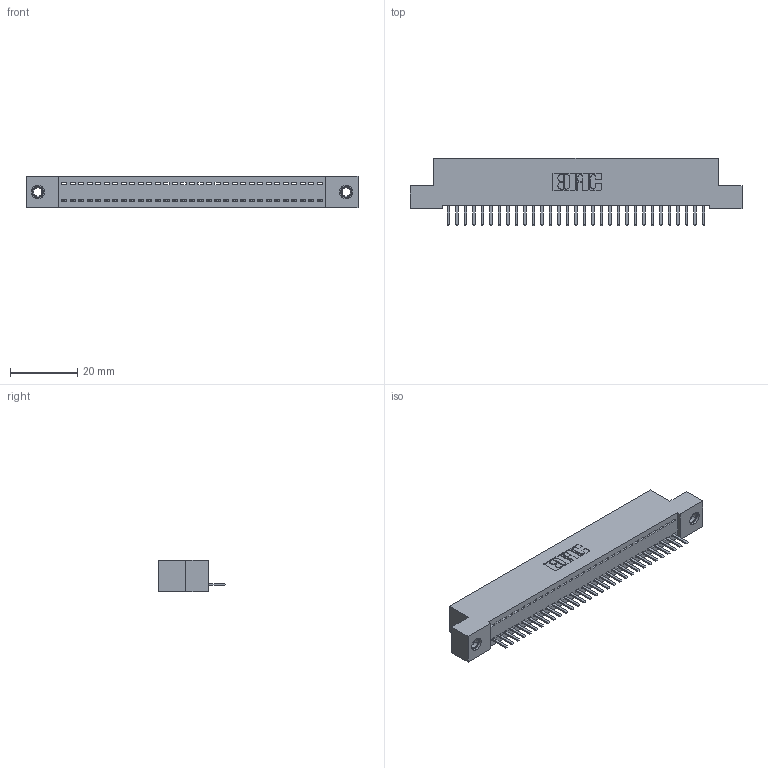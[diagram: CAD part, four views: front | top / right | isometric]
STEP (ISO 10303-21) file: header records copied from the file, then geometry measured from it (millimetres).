
FILE_DESCRIPTION (( 'STEP AP203' ), '1' );
FILE_NAME ('392-031-520-107.STEP', '2019-10-07T13:55:43', ( '' ), ( '' ), 'SwSTEP 2.0', 'SolidWorks 2016', '' );
FILE_SCHEMA (( 'CONFIG_CONTROL_DESIGN' ));
Length unit declared in the file: inch
Products named in the file (4): 345-292-001_345-293-120; 345-250-001_345-250-005-103; 392-031-520-107; 342 Part_TI
Assembly tree (34 placements, depth 2):
  392-031-520-107
    342 Part_TI
    345-292-001_345-293-120  x31
    345-250-001_345-250-005-103  x2
Bounding box: 99.06 x 20.02 x 9.4 mm (x, y, z)
Volume: 8543.2 mm3; surface area: 12086.9 mm2
Topology: 34 solids, 34 shells, 2092 faces, 6139 edges, 4002 vertices
Faces by surface type: plane 1462, cylinder 614, cone 12, torus 4
Entity records: 21542 total; most frequent: CARTESIAN_POINT 3710, ORIENTED_EDGE 3658, DIRECTION 3173, EDGE_CURVE 1829, LINE 1677, VECTOR 1677, VERTEX_POINT 1212, AXIS2_PLACEMENT_3D 748
